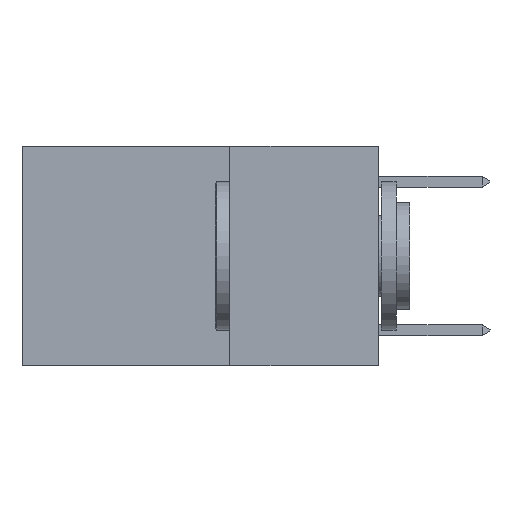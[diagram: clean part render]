
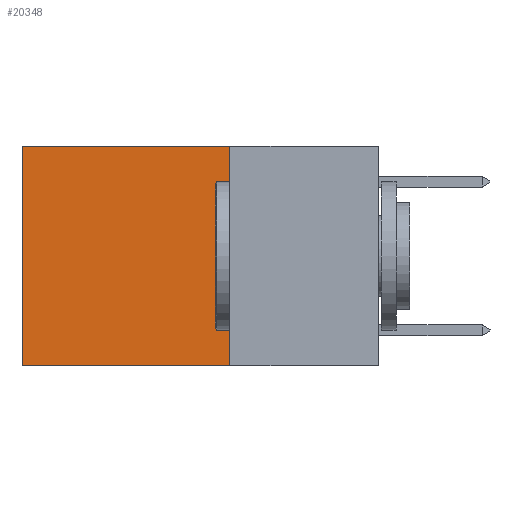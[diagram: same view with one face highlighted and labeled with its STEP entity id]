
A CAD part, left-side view. The second image highlights one B-rep face of the part: STEP entity #20348.
In plain terms, the highlighted planar face has unit normal (-1, 0, 0).
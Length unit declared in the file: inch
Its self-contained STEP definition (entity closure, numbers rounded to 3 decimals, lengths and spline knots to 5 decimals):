
#599 = EDGE_CURVE ( 'NONE', #11445, #20183, #5233, .T. ) ;
#900 = PLANE ( 'NONE',  #5088 ) ;
#1690 = CARTESIAN_POINT ( 'NONE',  ( 0.2625, 0.25, 0. ) ) ;
#2038 = VECTOR ( 'NONE', #21740, 39.37008 ) ;
#2208 = LINE ( 'NONE', #11438, #2038 ) ;
#2225 = DIRECTION ( 'NONE',  ( 1., 0., 0. ) ) ;
#3387 = VERTEX_POINT ( 'NONE', #21953 ) ;
#4324 = CARTESIAN_POINT ( 'NONE',  ( 0.2625, 0.25, -0.37 ) ) ;
#4668 = DIRECTION ( 'NONE',  ( 0., 0., -1. ) ) ;
#5088 = AXIS2_PLACEMENT_3D ( 'NONE', #20673, #2225, #9096 ) ;
#5233 = LINE ( 'NONE', #8271, #5352 ) ;
#5352 = VECTOR ( 'NONE', #8022, 39.37008 ) ;
#6314 = ORIENTED_EDGE ( 'NONE', *, *, #17245, .T. ) ;
#7697 = VERTEX_POINT ( 'NONE', #17467 ) ;
#8022 = DIRECTION ( 'NONE',  ( 0., 0., -1. ) ) ;
#8119 = EDGE_CURVE ( 'NONE', #20183, #3387, #2208, .T. ) ;
#8271 = CARTESIAN_POINT ( 'NONE',  ( 0.2625, 0.25, 0. ) ) ;
#9096 = DIRECTION ( 'NONE',  ( 0., 0., -1. ) ) ;
#9563 = ORIENTED_EDGE ( 'NONE', *, *, #19592, .T. ) ;
#10359 = LINE ( 'NONE', #1690, #10408 ) ;
#10408 = VECTOR ( 'NONE', #14425, 39.37008 ) ;
#11438 = CARTESIAN_POINT ( 'NONE',  ( 0.2625, 0.25, -0.37 ) ) ;
#11445 = VERTEX_POINT ( 'NONE', #17556 ) ;
#11559 = EDGE_LOOP ( 'NONE', ( #9563, #17165, #19523, #6314 ) ) ;
#11678 = FACE_OUTER_BOUND ( 'NONE', #11559, .T. ) ;
#14425 = DIRECTION ( 'NONE',  ( 0., 1., 0. ) ) ;
#17165 = ORIENTED_EDGE ( 'NONE', *, *, #8119, .F. ) ;
#17245 = EDGE_CURVE ( 'NONE', #11445, #7697, #10359, .T. ) ;
#17467 = CARTESIAN_POINT ( 'NONE',  ( 0.2625, 0.6, 0. ) ) ;
#17515 = VECTOR ( 'NONE', #4668, 39.37008 ) ;
#17556 = CARTESIAN_POINT ( 'NONE',  ( 0.2625, 0.25, 0. ) ) ;
#17781 = LINE ( 'NONE', #20634, #17515 ) ;
#19523 = ORIENTED_EDGE ( 'NONE', *, *, #599, .F. ) ;
#19592 = EDGE_CURVE ( 'NONE', #7697, #3387, #17781, .T. ) ;
#20183 = VERTEX_POINT ( 'NONE', #4324 ) ;
#20348 = ADVANCED_FACE ( 'NONE', ( #11678 ), #900, .F. ) ;
#20634 = CARTESIAN_POINT ( 'NONE',  ( 0.2625, 0.6, 0. ) ) ;
#20673 = CARTESIAN_POINT ( 'NONE',  ( 0.2625, 0.25, 0. ) ) ;
#21740 = DIRECTION ( 'NONE',  ( 0., 1., 0. ) ) ;
#21953 = CARTESIAN_POINT ( 'NONE',  ( 0.2625, 0.6, -0.37 ) ) ;
